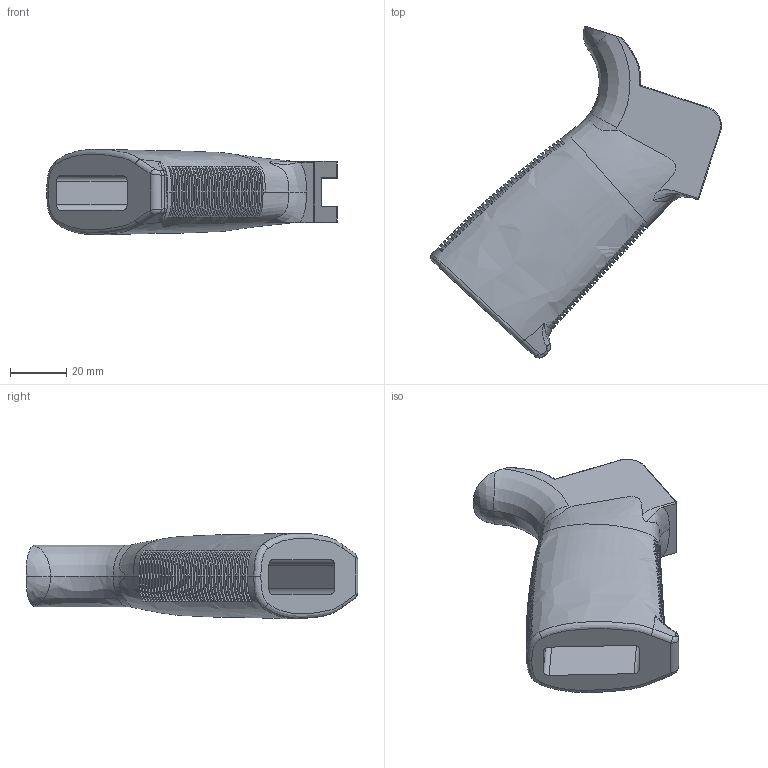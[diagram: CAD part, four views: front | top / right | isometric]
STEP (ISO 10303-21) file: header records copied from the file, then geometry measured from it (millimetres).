
FILE_DESCRIPTION (( 'STEP AP203' ), '1' );
FILE_NAME ('MP5 STYLE AR15 GRIP.STEP', '2020-09-02T22:00:13', ( '' ), ( '' ), 'SwSTEP 2.0', 'SolidWorks 2019', '' );
FILE_SCHEMA (( 'CONFIG_CONTROL_DESIGN' ));
Length unit declared in the file: centimetre
Products named in the file (1): MP5 STYLE AR15 GRIP
Bounding box: 103 x 117.6 x 30.18 mm (x, y, z)
Volume: 79771.7 mm3; surface area: 26370.5 mm2
Topology: 1 solids, 1 shells, 513 faces, 1481 edges, 968 vertices
Faces by surface type: plane 273, bspline 156, cylinder 54, torus 20, sphere 10
Entity records: 51260 total; most frequent: CARTESIAN_POINT 39526, ORIENTED_EDGE 2950, DIRECTION 1705, EDGE_CURVE 1475, VERTEX_POINT 966, B_SPLINE_CURVE_WITH_KNOTS 752, AXIS2_PLACEMENT_3D 643, EDGE_LOOP 517
